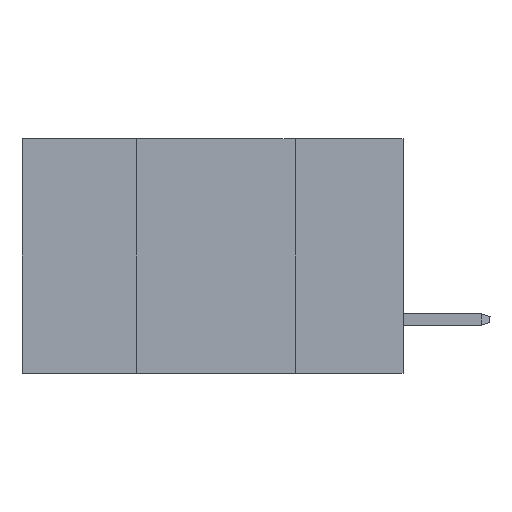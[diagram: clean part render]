
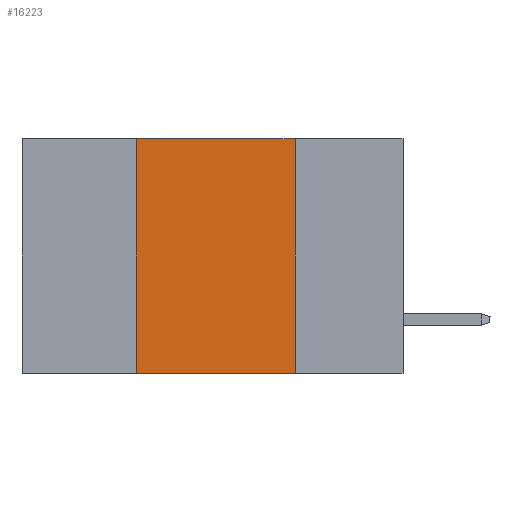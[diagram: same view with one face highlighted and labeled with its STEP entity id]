
A CAD part, left-side view. The second image highlights one B-rep face of the part: STEP entity #16223.
In plain terms, the highlighted planar face has unit normal (-1, 0, 0).
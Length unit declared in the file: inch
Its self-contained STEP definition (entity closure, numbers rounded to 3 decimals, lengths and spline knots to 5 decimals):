
#1475 = VECTOR ( 'NONE', #6426, 39.37008 ) ;
#2590 = DIRECTION ( 'NONE',  ( 1., 0., 0. ) ) ;
#2645 = DIRECTION ( 'NONE',  ( 0., -1., 0. ) ) ;
#3652 = VERTEX_POINT ( 'NONE', #24978 ) ;
#3867 = CARTESIAN_POINT ( 'NONE',  ( 0., 0.17, -0.37 ) ) ;
#4217 = LINE ( 'NONE', #8626, #1475 ) ;
#4234 = CARTESIAN_POINT ( 'NONE',  ( 0., 0.17, 0. ) ) ;
#4364 = LINE ( 'NONE', #4234, #23608 ) ;
#4554 = PLANE ( 'NONE',  #9423 ) ;
#4563 = ORIENTED_EDGE ( 'NONE', *, *, #24432, .T. ) ;
#5983 = EDGE_CURVE ( 'NONE', #16070, #3652, #13454, .T. ) ;
#6426 = DIRECTION ( 'NONE',  ( 0., -1., 0. ) ) ;
#6913 = CARTESIAN_POINT ( 'NONE',  ( 0., 0.6, 0. ) ) ;
#6990 = ORIENTED_EDGE ( 'NONE', *, *, #17852, .F. ) ;
#7629 = CARTESIAN_POINT ( 'NONE',  ( 0., 0.17, 0. ) ) ;
#7936 = EDGE_CURVE ( 'NONE', #9053, #16041, #4364, .T. ) ;
#8626 = CARTESIAN_POINT ( 'NONE',  ( 0., 0.6, 0. ) ) ;
#9053 = VERTEX_POINT ( 'NONE', #7629 ) ;
#9423 = AXIS2_PLACEMENT_3D ( 'NONE', #6913, #2590, #23570 ) ;
#10593 = VECTOR ( 'NONE', #11764, 39.37008 ) ;
#11679 = LINE ( 'NONE', #17937, #19879 ) ;
#11764 = DIRECTION ( 'NONE',  ( 0., 0., 1. ) ) ;
#13454 = LINE ( 'NONE', #21918, #10593 ) ;
#16041 = VERTEX_POINT ( 'NONE', #3867 ) ;
#16070 = VERTEX_POINT ( 'NONE', #24949 ) ;
#16223 = ADVANCED_FACE ( 'NONE', ( #23419 ), #4554, .F. ) ;
#17852 = EDGE_CURVE ( 'NONE', #3652, #9053, #4217, .T. ) ;
#17937 = CARTESIAN_POINT ( 'NONE',  ( 0., 0.6, -0.37 ) ) ;
#19879 = VECTOR ( 'NONE', #2645, 39.37008 ) ;
#20383 = ORIENTED_EDGE ( 'NONE', *, *, #5983, .F. ) ;
#21918 = CARTESIAN_POINT ( 'NONE',  ( 0., 0.42, 0. ) ) ;
#23419 = FACE_OUTER_BOUND ( 'NONE', #26509, .T. ) ;
#23570 = DIRECTION ( 'NONE',  ( 0., 0., -1. ) ) ;
#23608 = VECTOR ( 'NONE', #25595, 39.37008 ) ;
#23968 = ORIENTED_EDGE ( 'NONE', *, *, #7936, .F. ) ;
#24432 = EDGE_CURVE ( 'NONE', #16070, #16041, #11679, .T. ) ;
#24949 = CARTESIAN_POINT ( 'NONE',  ( 0., 0.42, -0.37 ) ) ;
#24978 = CARTESIAN_POINT ( 'NONE',  ( 0., 0.42, 0. ) ) ;
#25595 = DIRECTION ( 'NONE',  ( 0., 0., -1. ) ) ;
#26509 = EDGE_LOOP ( 'NONE', ( #23968, #6990, #20383, #4563 ) ) ;
